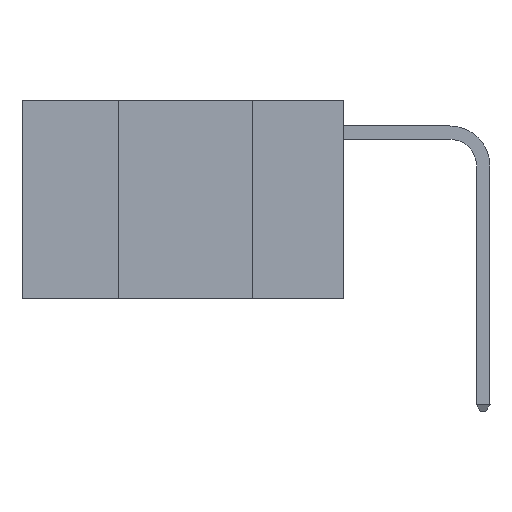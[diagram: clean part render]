
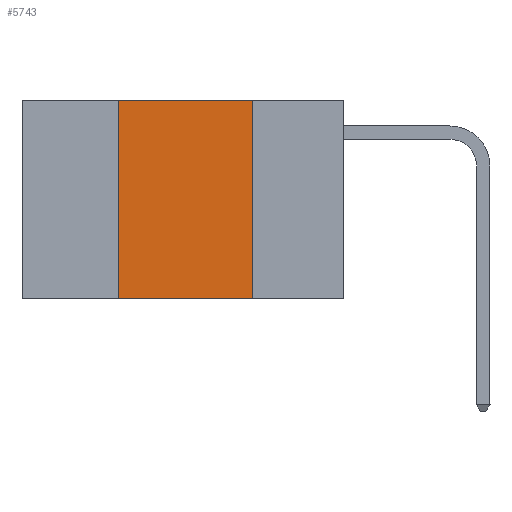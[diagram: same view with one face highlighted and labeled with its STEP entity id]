
A CAD part, left-side view. The second image highlights one B-rep face of the part: STEP entity #5743.
In plain terms, the highlighted planar face has unit normal (-1, 0, 0).
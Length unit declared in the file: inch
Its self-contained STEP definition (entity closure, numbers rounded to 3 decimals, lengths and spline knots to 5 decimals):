
#590 = LINE ( 'NONE', #13317, #15418 ) ;
#939 = VERTEX_POINT ( 'NONE', #1973 ) ;
#1961 = LINE ( 'NONE', #12533, #16727 ) ;
#1973 = CARTESIAN_POINT ( 'NONE',  ( 0., 0.17, -0.37 ) ) ;
#2051 = ORIENTED_EDGE ( 'NONE', *, *, #16716, .T. ) ;
#2447 = VECTOR ( 'NONE', #15062, 39.37008 ) ;
#2908 = LINE ( 'NONE', #12290, #2447 ) ;
#4148 = DIRECTION ( 'NONE',  ( 0., 0., -1. ) ) ;
#4318 = ORIENTED_EDGE ( 'NONE', *, *, #4717, .F. ) ;
#4717 = EDGE_CURVE ( 'NONE', #11199, #11014, #1961, .T. ) ;
#5743 = ADVANCED_FACE ( 'NONE', ( #11214 ), #9908, .F. ) ;
#5773 = DIRECTION ( 'NONE',  ( 0., -1., 0. ) ) ;
#6864 = EDGE_CURVE ( 'NONE', #11014, #939, #2908, .T. ) ;
#7067 = VECTOR ( 'NONE', #5773, 39.37008 ) ;
#7842 = EDGE_CURVE ( 'NONE', #16005, #11199, #590, .T. ) ;
#8444 = CARTESIAN_POINT ( 'NONE',  ( 0., 0.42, -0.37 ) ) ;
#9081 = LINE ( 'NONE', #14319, #7067 ) ;
#9908 = PLANE ( 'NONE',  #17432 ) ;
#11014 = VERTEX_POINT ( 'NONE', #15678 ) ;
#11199 = VERTEX_POINT ( 'NONE', #11572 ) ;
#11214 = FACE_OUTER_BOUND ( 'NONE', #15771, .T. ) ;
#11359 = CARTESIAN_POINT ( 'NONE',  ( 0., 0.6, 0. ) ) ;
#11572 = CARTESIAN_POINT ( 'NONE',  ( 0., 0.42, 0. ) ) ;
#12290 = CARTESIAN_POINT ( 'NONE',  ( 0., 0.17, 0. ) ) ;
#12533 = CARTESIAN_POINT ( 'NONE',  ( 0., 0.6, 0. ) ) ;
#12762 = DIRECTION ( 'NONE',  ( 1., 0., 0. ) ) ;
#13317 = CARTESIAN_POINT ( 'NONE',  ( 0., 0.42, 0. ) ) ;
#14319 = CARTESIAN_POINT ( 'NONE',  ( 0., 0.6, -0.37 ) ) ;
#14854 = ORIENTED_EDGE ( 'NONE', *, *, #7842, .F. ) ;
#15062 = DIRECTION ( 'NONE',  ( 0., 0., -1. ) ) ;
#15069 = ORIENTED_EDGE ( 'NONE', *, *, #6864, .F. ) ;
#15361 = DIRECTION ( 'NONE',  ( 0., -1., 0. ) ) ;
#15418 = VECTOR ( 'NONE', #16139, 39.37008 ) ;
#15678 = CARTESIAN_POINT ( 'NONE',  ( 0., 0.17, 0. ) ) ;
#15771 = EDGE_LOOP ( 'NONE', ( #15069, #4318, #14854, #2051 ) ) ;
#16005 = VERTEX_POINT ( 'NONE', #8444 ) ;
#16139 = DIRECTION ( 'NONE',  ( 0., 0., 1. ) ) ;
#16716 = EDGE_CURVE ( 'NONE', #16005, #939, #9081, .T. ) ;
#16727 = VECTOR ( 'NONE', #15361, 39.37008 ) ;
#17432 = AXIS2_PLACEMENT_3D ( 'NONE', #11359, #12762, #4148 ) ;
